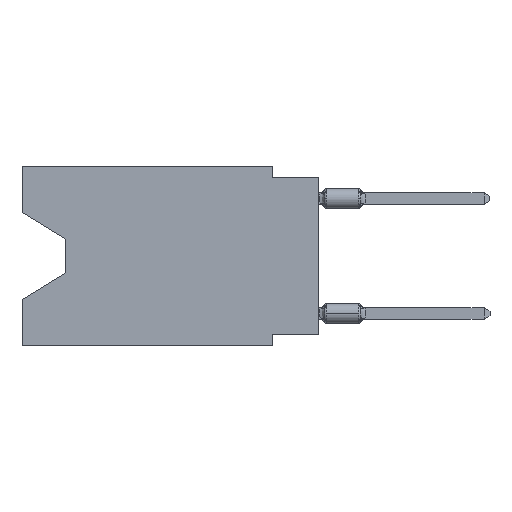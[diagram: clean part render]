
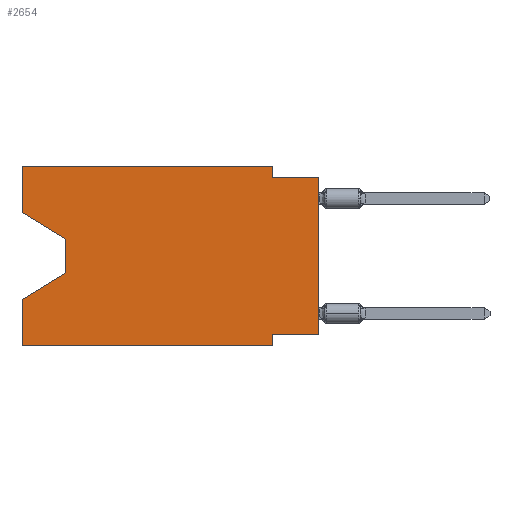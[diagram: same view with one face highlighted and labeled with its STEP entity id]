
A CAD part, left-side view. The second image highlights one B-rep face of the part: STEP entity #2654.
In plain terms, the highlighted planar face has unit normal (-1, 0, 0).
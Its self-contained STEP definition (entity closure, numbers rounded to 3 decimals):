
#47 = VECTOR ( 'NONE', #3817, 1000. ) ;
#485 = ORIENTED_EDGE ( 'NONE', *, *, #7329, .F. ) ;
#587 = CARTESIAN_POINT ( 'NONE',  ( 0., 0., -9.271 ) ) ;
#906 = EDGE_CURVE ( 'NONE', #5066, #6735, #11756, .T. ) ;
#907 = EDGE_CURVE ( 'NONE', #4599, #4208, #5812, .T. ) ;
#953 = EDGE_CURVE ( 'NONE', #6848, #11554, #6252, .T. ) ;
#1092 = VERTEX_POINT ( 'NONE', #2346 ) ;
#1121 = DIRECTION ( 'NONE',  ( 0., 0.855, -0.519 ) ) ;
#1245 = LINE ( 'NONE', #10122, #5499 ) ;
#1273 = DIRECTION ( 'NONE',  ( 0., 0., -1. ) ) ;
#1418 = LINE ( 'NONE', #3323, #3668 ) ;
#1479 = DIRECTION ( 'NONE',  ( 0., 0., -1. ) ) ;
#1637 = EDGE_CURVE ( 'NONE', #4208, #5134, #1245, .T. ) ;
#1776 = DIRECTION ( 'NONE',  ( 0., -1., 0. ) ) ;
#2025 = CARTESIAN_POINT ( 'NONE',  ( 0., 16.383, 0. ) ) ;
#2346 = CARTESIAN_POINT ( 'NONE',  ( 0., 16.383, -2.546 ) ) ;
#2358 = DIRECTION ( 'NONE',  ( 0., 0., 1. ) ) ;
#2654 = ADVANCED_FACE ( 'NONE', ( #4324 ), #6293, .F. ) ;
#2737 = ORIENTED_EDGE ( 'NONE', *, *, #4322, .T. ) ;
#2750 = VERTEX_POINT ( 'NONE', #3786 ) ;
#2858 = VECTOR ( 'NONE', #6908, 1000. ) ;
#3226 = ORIENTED_EDGE ( 'NONE', *, *, #7841, .F. ) ;
#3323 = CARTESIAN_POINT ( 'NONE',  ( 0., 2.54, -9.906 ) ) ;
#3344 = CARTESIAN_POINT ( 'NONE',  ( 0., 13.97, -4.013 ) ) ;
#3668 = VECTOR ( 'NONE', #1479, 1000. ) ;
#3683 = LINE ( 'NONE', #587, #10795 ) ;
#3707 = VECTOR ( 'NONE', #12593, 1000. ) ;
#3786 = CARTESIAN_POINT ( 'NONE',  ( 0., 0., -0.635 ) ) ;
#3787 = CARTESIAN_POINT ( 'NONE',  ( 0., 16.383, 0. ) ) ;
#3817 = DIRECTION ( 'NONE',  ( 0., 0., -1. ) ) ;
#3828 = LINE ( 'NONE', #12088, #2858 ) ;
#4007 = VECTOR ( 'NONE', #4695, 1000. ) ;
#4025 = VECTOR ( 'NONE', #7033, 1000. ) ;
#4096 = VECTOR ( 'NONE', #2358, 1000. ) ;
#4208 = VERTEX_POINT ( 'NONE', #11454 ) ;
#4322 = EDGE_CURVE ( 'NONE', #1092, #4599, #10662, .T. ) ;
#4324 = FACE_OUTER_BOUND ( 'NONE', #8085, .T. ) ;
#4599 = VERTEX_POINT ( 'NONE', #3344 ) ;
#4695 = DIRECTION ( 'NONE',  ( 0., -0.855, -0.519 ) ) ;
#4792 = EDGE_CURVE ( 'NONE', #1092, #5066, #4995, .T. ) ;
#4947 = ORIENTED_EDGE ( 'NONE', *, *, #10070, .F. ) ;
#4969 = CARTESIAN_POINT ( 'NONE',  ( 0., 16.383, -9.906 ) ) ;
#4995 = LINE ( 'NONE', #2025, #8423 ) ;
#5056 = DIRECTION ( 'NONE',  ( 0., 0., 1. ) ) ;
#5066 = VERTEX_POINT ( 'NONE', #3787 ) ;
#5134 = VERTEX_POINT ( 'NONE', #7859 ) ;
#5331 = CARTESIAN_POINT ( 'NONE',  ( 0., 0., 0. ) ) ;
#5499 = VECTOR ( 'NONE', #1121, 1000. ) ;
#5652 = CARTESIAN_POINT ( 'NONE',  ( 0., 16.383, 0. ) ) ;
#5667 = ORIENTED_EDGE ( 'NONE', *, *, #8319, .T. ) ;
#5673 = ORIENTED_EDGE ( 'NONE', *, *, #906, .F. ) ;
#5779 = LINE ( 'NONE', #6558, #6199 ) ;
#5812 = LINE ( 'NONE', #5871, #47 ) ;
#5834 = CARTESIAN_POINT ( 'NONE',  ( 0., 2.54, 0. ) ) ;
#5871 = CARTESIAN_POINT ( 'NONE',  ( 0., 13.97, -4.013 ) ) ;
#5937 = ORIENTED_EDGE ( 'NONE', *, *, #7583, .F. ) ;
#6062 = CARTESIAN_POINT ( 'NONE',  ( 0., 16.383, -9.906 ) ) ;
#6129 = CARTESIAN_POINT ( 'NONE',  ( 0., 2.54, -0.635 ) ) ;
#6152 = AXIS2_PLACEMENT_3D ( 'NONE', #9432, #6492, #1273 ) ;
#6199 = VECTOR ( 'NONE', #7531, 1000. ) ;
#6228 = ORIENTED_EDGE ( 'NONE', *, *, #4792, .F. ) ;
#6252 = LINE ( 'NONE', #6062, #4025 ) ;
#6293 = PLANE ( 'NONE',  #6152 ) ;
#6492 = DIRECTION ( 'NONE',  ( 1., 0., 0. ) ) ;
#6558 = CARTESIAN_POINT ( 'NONE',  ( 0., 2.54, 0. ) ) ;
#6735 = VERTEX_POINT ( 'NONE', #5834 ) ;
#6848 = VERTEX_POINT ( 'NONE', #4969 ) ;
#6908 = DIRECTION ( 'NONE',  ( 0., -1., 0. ) ) ;
#7033 = DIRECTION ( 'NONE',  ( 0., -1., 0. ) ) ;
#7224 = LINE ( 'NONE', #5331, #4096 ) ;
#7329 = EDGE_CURVE ( 'NONE', #8254, #2750, #3828, .T. ) ;
#7531 = DIRECTION ( 'NONE',  ( 0., 0., -1. ) ) ;
#7583 = EDGE_CURVE ( 'NONE', #10894, #9799, #3683, .T. ) ;
#7690 = DIRECTION ( 'NONE',  ( 0., 1., 0. ) ) ;
#7841 = EDGE_CURVE ( 'NONE', #6735, #8254, #5779, .T. ) ;
#7859 = CARTESIAN_POINT ( 'NONE',  ( 0., 16.383, -7.36 ) ) ;
#8085 = EDGE_LOOP ( 'NONE', ( #2737, #9444, #12521, #4947, #9239, #8391, #5937, #5667, #485, #3226, #5673, #6228 ) ) ;
#8254 = VERTEX_POINT ( 'NONE', #6129 ) ;
#8319 = EDGE_CURVE ( 'NONE', #10894, #2750, #7224, .T. ) ;
#8391 = ORIENTED_EDGE ( 'NONE', *, *, #11518, .F. ) ;
#8423 = VECTOR ( 'NONE', #5056, 1000. ) ;
#8802 = CARTESIAN_POINT ( 'NONE',  ( 0., 16.383, 0. ) ) ;
#8812 = CARTESIAN_POINT ( 'NONE',  ( 0., 0., -9.271 ) ) ;
#8845 = LINE ( 'NONE', #5652, #3707 ) ;
#9239 = ORIENTED_EDGE ( 'NONE', *, *, #953, .T. ) ;
#9432 = CARTESIAN_POINT ( 'NONE',  ( 0., 16.383, 0. ) ) ;
#9444 = ORIENTED_EDGE ( 'NONE', *, *, #907, .T. ) ;
#9799 = VERTEX_POINT ( 'NONE', #11218 ) ;
#10070 = EDGE_CURVE ( 'NONE', #6848, #5134, #8845, .T. ) ;
#10122 = CARTESIAN_POINT ( 'NONE',  ( 0., 13.97, -5.893 ) ) ;
#10593 = CARTESIAN_POINT ( 'NONE',  ( 0., 16.383, -2.546 ) ) ;
#10662 = LINE ( 'NONE', #10593, #4007 ) ;
#10795 = VECTOR ( 'NONE', #7690, 1000. ) ;
#10894 = VERTEX_POINT ( 'NONE', #8812 ) ;
#11218 = CARTESIAN_POINT ( 'NONE',  ( 0., 2.54, -9.271 ) ) ;
#11454 = CARTESIAN_POINT ( 'NONE',  ( 0., 13.97, -5.893 ) ) ;
#11518 = EDGE_CURVE ( 'NONE', #9799, #11554, #1418, .T. ) ;
#11554 = VERTEX_POINT ( 'NONE', #12317 ) ;
#11756 = LINE ( 'NONE', #8802, #11969 ) ;
#11969 = VECTOR ( 'NONE', #1776, 1000. ) ;
#12088 = CARTESIAN_POINT ( 'NONE',  ( 0., 0., -0.635 ) ) ;
#12317 = CARTESIAN_POINT ( 'NONE',  ( 0., 2.54, -9.906 ) ) ;
#12521 = ORIENTED_EDGE ( 'NONE', *, *, #1637, .T. ) ;
#12593 = DIRECTION ( 'NONE',  ( 0., 0., 1. ) ) ;
